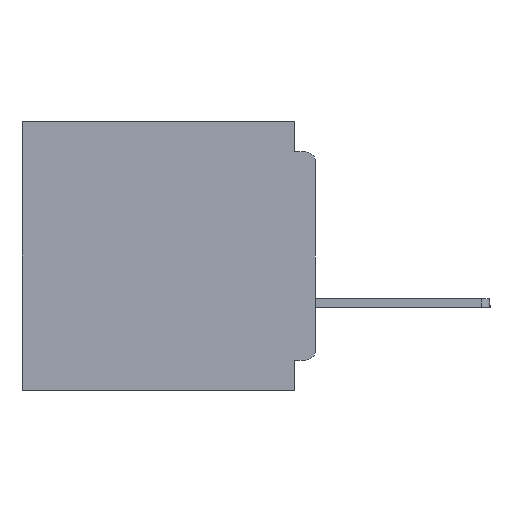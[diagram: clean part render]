
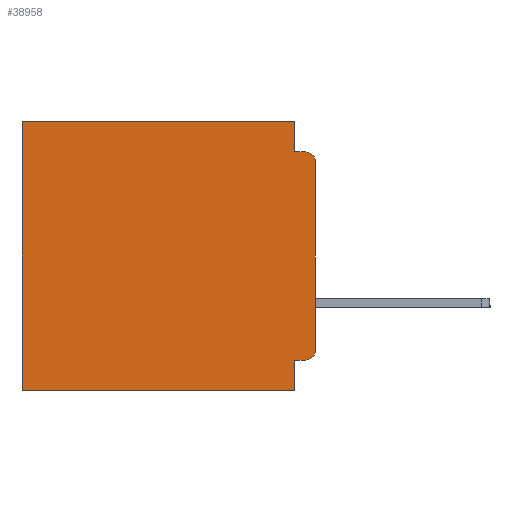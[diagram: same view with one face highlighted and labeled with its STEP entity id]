
A CAD part, left-side view. The second image highlights one B-rep face of the part: STEP entity #38958.
In plain terms, the highlighted planar face has unit normal (-1, 0, 0).
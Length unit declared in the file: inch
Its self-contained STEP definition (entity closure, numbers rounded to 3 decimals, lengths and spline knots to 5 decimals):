
#79 = LINE ( 'NONE', #40806, #43082 ) ;
#214 = AXIS2_PLACEMENT_3D ( 'NONE', #9307, #19576, #43187 ) ;
#1067 = CARTESIAN_POINT ( 'NONE',  ( 0.3, 0.031, -0.4 ) ) ;
#1477 = DIRECTION ( 'NONE',  ( -1., 0., 0. ) ) ;
#2025 = CARTESIAN_POINT ( 'NONE',  ( 0.3, 0.031, 0. ) ) ;
#2123 = ORIENTED_EDGE ( 'NONE', *, *, #7475, .T. ) ;
#2257 = VERTEX_POINT ( 'NONE', #13610 ) ;
#2278 = CARTESIAN_POINT ( 'NONE',  ( 0.3, 0., -0.4 ) ) ;
#3098 = CARTESIAN_POINT ( 'NONE',  ( 0.3, 0.031, -0.4 ) ) ;
#3181 = VECTOR ( 'NONE', #3960, 39.37008 ) ;
#3724 = CARTESIAN_POINT ( 'NONE',  ( 0.3, 0.031, -0.045 ) ) ;
#3814 = EDGE_CURVE ( 'NONE', #9900, #28170, #15489, .T. ) ;
#3960 = DIRECTION ( 'NONE',  ( 0., 1., 0. ) ) ;
#4040 = AXIS2_PLACEMENT_3D ( 'NONE', #15416, #39111, #18815 ) ;
#4105 = VERTEX_POINT ( 'NONE', #18401 ) ;
#4266 = LINE ( 'NONE', #14136, #3181 ) ;
#4396 = EDGE_CURVE ( 'NONE', #9589, #2257, #43927, .T. ) ;
#7190 = LINE ( 'NONE', #16198, #33342 ) ;
#7475 = EDGE_CURVE ( 'NONE', #33680, #9900, #4266, .T. ) ;
#7803 = EDGE_CURVE ( 'NONE', #16005, #28170, #17577, .T. ) ;
#8043 = ORIENTED_EDGE ( 'NONE', *, *, #26977, .F. ) ;
#9140 = DIRECTION ( 'NONE',  ( 0., 1., 0. ) ) ;
#9307 = CARTESIAN_POINT ( 'NONE',  ( 0.3, 0., -0.4 ) ) ;
#9589 = VERTEX_POINT ( 'NONE', #18833 ) ;
#9900 = VERTEX_POINT ( 'NONE', #20559 ) ;
#10447 = LINE ( 'NONE', #1067, #19490 ) ;
#11242 = ORIENTED_EDGE ( 'NONE', *, *, #7803, .F. ) ;
#11759 = ORIENTED_EDGE ( 'NONE', *, *, #3814, .T. ) ;
#12768 = PLANE ( 'NONE',  #214 ) ;
#12820 = ORIENTED_EDGE ( 'NONE', *, *, #42994, .F. ) ;
#13610 = CARTESIAN_POINT ( 'NONE',  ( 0.3, 0.031, -0.355 ) ) ;
#14136 = CARTESIAN_POINT ( 'NONE',  ( 0.3, 0., 0. ) ) ;
#14889 = CIRCLE ( 'NONE', #4040, 0.015 ) ;
#15416 = CARTESIAN_POINT ( 'NONE',  ( 0.3, 0.015, -0.06 ) ) ;
#15489 = LINE ( 'NONE', #19833, #40377 ) ;
#16005 = VERTEX_POINT ( 'NONE', #3098 ) ;
#16198 = CARTESIAN_POINT ( 'NONE',  ( 0.3, 0.031, 0. ) ) ;
#17577 = LINE ( 'NONE', #2278, #34631 ) ;
#17979 = CIRCLE ( 'NONE', #18937, 0.015 ) ;
#18076 = VECTOR ( 'NONE', #42645, 39.37008 ) ;
#18401 = CARTESIAN_POINT ( 'NONE',  ( 0.3, 0.015, -0.045 ) ) ;
#18470 = VECTOR ( 'NONE', #20461, 39.37008 ) ;
#18815 = DIRECTION ( 'NONE',  ( 0., 0., -1. ) ) ;
#18833 = CARTESIAN_POINT ( 'NONE',  ( 0.3, 0.015, -0.355 ) ) ;
#18937 = AXIS2_PLACEMENT_3D ( 'NONE', #21922, #1477, #25362 ) ;
#19490 = VECTOR ( 'NONE', #28426, 39.37008 ) ;
#19576 = DIRECTION ( 'NONE',  ( 1., 0., 0. ) ) ;
#19833 = CARTESIAN_POINT ( 'NONE',  ( 0.3, 0.437, -0.4 ) ) ;
#20365 = EDGE_CURVE ( 'NONE', #22646, #4105, #79, .T. ) ;
#20461 = DIRECTION ( 'NONE',  ( 0., 0., -1. ) ) ;
#20559 = CARTESIAN_POINT ( 'NONE',  ( 0.3, 0.437, 0. ) ) ;
#20679 = DIRECTION ( 'NONE',  ( 0., -1., 0. ) ) ;
#20829 = CARTESIAN_POINT ( 'NONE',  ( 0.3, 0.437, -0.4 ) ) ;
#21922 = CARTESIAN_POINT ( 'NONE',  ( 0.3, 0.015, -0.34 ) ) ;
#22646 = VERTEX_POINT ( 'NONE', #3724 ) ;
#23044 = ORIENTED_EDGE ( 'NONE', *, *, #33781, .F. ) ;
#23954 = CARTESIAN_POINT ( 'NONE',  ( 0.3, 0., -0.4 ) ) ;
#24037 = ORIENTED_EDGE ( 'NONE', *, *, #20365, .F. ) ;
#25031 = FACE_OUTER_BOUND ( 'NONE', #33349, .T. ) ;
#25362 = DIRECTION ( 'NONE',  ( 0., 0., -1. ) ) ;
#25604 = VERTEX_POINT ( 'NONE', #27789 ) ;
#26977 = EDGE_CURVE ( 'NONE', #2257, #16005, #10447, .T. ) ;
#27789 = CARTESIAN_POINT ( 'NONE',  ( 0.3, 0., -0.06 ) ) ;
#27994 = DIRECTION ( 'NONE',  ( 0., 0., -1. ) ) ;
#28170 = VERTEX_POINT ( 'NONE', #20829 ) ;
#28426 = DIRECTION ( 'NONE',  ( 0., 0., -1. ) ) ;
#30372 = CARTESIAN_POINT ( 'NONE',  ( 0.3, 0., -0.34 ) ) ;
#30933 = ORIENTED_EDGE ( 'NONE', *, *, #41622, .T. ) ;
#31525 = ORIENTED_EDGE ( 'NONE', *, *, #32675, .T. ) ;
#32675 = EDGE_CURVE ( 'NONE', #9589, #41215, #17979, .T. ) ;
#33342 = VECTOR ( 'NONE', #36555, 39.37008 ) ;
#33349 = EDGE_LOOP ( 'NONE', ( #12820, #30933, #24037, #23044, #2123, #11759, #11242, #8043, #43526, #31525 ) ) ;
#33680 = VERTEX_POINT ( 'NONE', #2025 ) ;
#33781 = EDGE_CURVE ( 'NONE', #33680, #22646, #7190, .T. ) ;
#34631 = VECTOR ( 'NONE', #9140, 39.37008 ) ;
#36535 = LINE ( 'NONE', #23954, #18470 ) ;
#36555 = DIRECTION ( 'NONE',  ( 0., 0., -1. ) ) ;
#38958 = ADVANCED_FACE ( 'NONE', ( #25031 ), #12768, .F. ) ;
#39111 = DIRECTION ( 'NONE',  ( -1., 0., 0. ) ) ;
#40377 = VECTOR ( 'NONE', #27994, 39.37008 ) ;
#40806 = CARTESIAN_POINT ( 'NONE',  ( 0.3, 0., -0.045 ) ) ;
#41215 = VERTEX_POINT ( 'NONE', #30372 ) ;
#41622 = EDGE_CURVE ( 'NONE', #25604, #4105, #14889, .T. ) ;
#42645 = DIRECTION ( 'NONE',  ( 0., 1., 0. ) ) ;
#42743 = CARTESIAN_POINT ( 'NONE',  ( 0.3, 0., -0.355 ) ) ;
#42994 = EDGE_CURVE ( 'NONE', #25604, #41215, #36535, .T. ) ;
#43082 = VECTOR ( 'NONE', #20679, 39.37008 ) ;
#43187 = DIRECTION ( 'NONE',  ( 0., 0., -1. ) ) ;
#43526 = ORIENTED_EDGE ( 'NONE', *, *, #4396, .F. ) ;
#43927 = LINE ( 'NONE', #42743, #18076 ) ;
